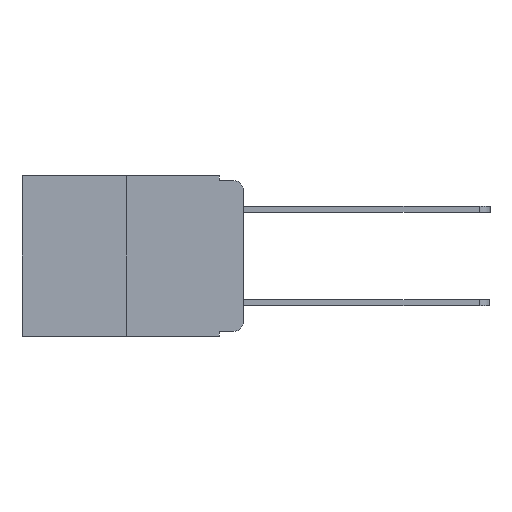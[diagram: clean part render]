
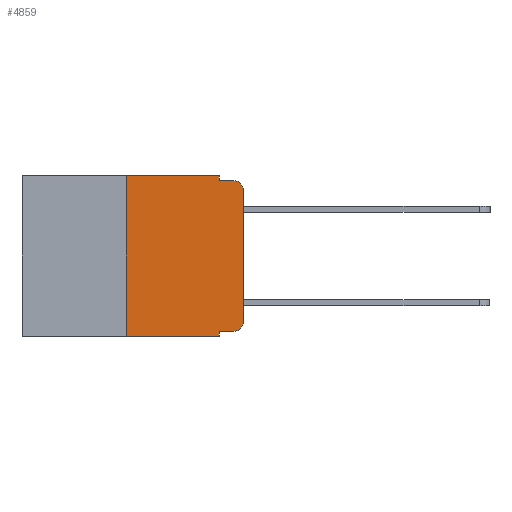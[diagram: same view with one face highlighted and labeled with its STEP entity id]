
A CAD part, left-side view. The second image highlights one B-rep face of the part: STEP entity #4859.
In plain terms, the highlighted planar face has unit normal (-1, 0, 0).
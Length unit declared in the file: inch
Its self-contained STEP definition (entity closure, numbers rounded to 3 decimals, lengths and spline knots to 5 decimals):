
#350 = VERTEX_POINT ( 'NONE', #8373 ) ;
#452 = LINE ( 'NONE', #888, #8284 ) ;
#463 = DIRECTION ( 'NONE',  ( 0., 0., -1. ) ) ;
#888 = CARTESIAN_POINT ( 'NONE',  ( 0., 0.473, -0.343 ) ) ;
#936 = CARTESIAN_POINT ( 'NONE',  ( 0., 0.051, -0.333 ) ) ;
#1066 = ORIENTED_EDGE ( 'NONE', *, *, #5062, .F. ) ;
#1341 = CIRCLE ( 'NONE', #8610, 0.02 ) ;
#1347 = PLANE ( 'NONE',  #12358 ) ;
#1623 = LINE ( 'NONE', #2709, #12249 ) ;
#1631 = CARTESIAN_POINT ( 'NONE',  ( 0., 0.02, -0.333 ) ) ;
#1975 = EDGE_CURVE ( 'NONE', #10013, #10409, #1341, .T. ) ;
#2271 = LINE ( 'NONE', #11626, #12430 ) ;
#2469 = CARTESIAN_POINT ( 'NONE',  ( 0., 0.02, -0.03 ) ) ;
#2486 = VECTOR ( 'NONE', #4466, 39.37008 ) ;
#2709 = CARTESIAN_POINT ( 'NONE',  ( 0., 0.25, 0. ) ) ;
#2778 = EDGE_CURVE ( 'NONE', #6278, #10013, #9922, .T. ) ;
#3010 = ORIENTED_EDGE ( 'NONE', *, *, #7052, .T. ) ;
#3374 = DIRECTION ( 'NONE',  ( 0., -1., 0. ) ) ;
#3494 = ORIENTED_EDGE ( 'NONE', *, *, #8105, .T. ) ;
#3567 = EDGE_CURVE ( 'NONE', #6278, #4012, #2271, .T. ) ;
#3633 = DIRECTION ( 'NONE',  ( 0., 0., -1. ) ) ;
#3638 = DIRECTION ( 'NONE',  ( 0., 0., -1. ) ) ;
#3853 = DIRECTION ( 'NONE',  ( 0., -1., 0. ) ) ;
#3870 = ORIENTED_EDGE ( 'NONE', *, *, #1975, .T. ) ;
#3961 = VECTOR ( 'NONE', #3853, 39.37008 ) ;
#4004 = CARTESIAN_POINT ( 'NONE',  ( 0., 0.051, -0.333 ) ) ;
#4012 = VERTEX_POINT ( 'NONE', #10223 ) ;
#4240 = EDGE_CURVE ( 'NONE', #5392, #350, #13506, .T. ) ;
#4338 = EDGE_CURVE ( 'NONE', #12383, #5392, #1623, .T. ) ;
#4466 = DIRECTION ( 'NONE',  ( 0., 0., 1. ) ) ;
#4538 = CARTESIAN_POINT ( 'NONE',  ( 0., 0.25, -0.343 ) ) ;
#4859 = ADVANCED_FACE ( 'NONE', ( #8910 ), #1347, .F. ) ;
#4999 = DIRECTION ( 'NONE',  ( 0., 0., 1. ) ) ;
#5062 = EDGE_CURVE ( 'NONE', #350, #11182, #11923, .T. ) ;
#5392 = VERTEX_POINT ( 'NONE', #8377 ) ;
#5452 = LINE ( 'NONE', #11368, #2486 ) ;
#5738 = EDGE_CURVE ( 'NONE', #11182, #8103, #9769, .T. ) ;
#5886 = CARTESIAN_POINT ( 'NONE',  ( 0., 0.473, 0. ) ) ;
#5915 = DIRECTION ( 'NONE',  ( 0., 0., -1. ) ) ;
#5934 = ORIENTED_EDGE ( 'NONE', *, *, #6382, .T. ) ;
#6021 = DIRECTION ( 'NONE',  ( -1., 0., 0. ) ) ;
#6278 = VERTEX_POINT ( 'NONE', #936 ) ;
#6300 = ORIENTED_EDGE ( 'NONE', *, *, #2778, .T. ) ;
#6382 = EDGE_CURVE ( 'NONE', #7345, #8103, #13264, .T. ) ;
#6808 = ORIENTED_EDGE ( 'NONE', *, *, #4338, .F. ) ;
#6817 = CARTESIAN_POINT ( 'NONE',  ( 0., 0., -0.03 ) ) ;
#7052 = EDGE_CURVE ( 'NONE', #10409, #7345, #5452, .T. ) ;
#7263 = ORIENTED_EDGE ( 'NONE', *, *, #4240, .F. ) ;
#7345 = VERTEX_POINT ( 'NONE', #6817 ) ;
#8103 = VERTEX_POINT ( 'NONE', #13322 ) ;
#8105 = EDGE_CURVE ( 'NONE', #12383, #4012, #452, .T. ) ;
#8147 = AXIS2_PLACEMENT_3D ( 'NONE', #2469, #9712, #3638 ) ;
#8284 = VECTOR ( 'NONE', #3374, 39.37008 ) ;
#8373 = CARTESIAN_POINT ( 'NONE',  ( 0., 0.051, 0. ) ) ;
#8377 = CARTESIAN_POINT ( 'NONE',  ( 0., 0.25, 0. ) ) ;
#8610 = AXIS2_PLACEMENT_3D ( 'NONE', #11833, #6021, #12823 ) ;
#8658 = CARTESIAN_POINT ( 'NONE',  ( 0., 0., -0.313 ) ) ;
#8910 = FACE_OUTER_BOUND ( 'NONE', #10729, .T. ) ;
#9351 = ORIENTED_EDGE ( 'NONE', *, *, #3567, .F. ) ;
#9361 = VECTOR ( 'NONE', #463, 39.37008 ) ;
#9456 = ORIENTED_EDGE ( 'NONE', *, *, #5738, .F. ) ;
#9462 = CARTESIAN_POINT ( 'NONE',  ( 0., 0.051, -0.01 ) ) ;
#9712 = DIRECTION ( 'NONE',  ( -1., 0., 0. ) ) ;
#9769 = LINE ( 'NONE', #10856, #3961 ) ;
#9812 = CARTESIAN_POINT ( 'NONE',  ( 0., 0.473, 0. ) ) ;
#9922 = LINE ( 'NONE', #4004, #10235 ) ;
#10013 = VERTEX_POINT ( 'NONE', #1631 ) ;
#10223 = CARTESIAN_POINT ( 'NONE',  ( 0., 0.051, -0.343 ) ) ;
#10235 = VECTOR ( 'NONE', #10986, 39.37008 ) ;
#10409 = VERTEX_POINT ( 'NONE', #8658 ) ;
#10729 = EDGE_LOOP ( 'NONE', ( #3010, #5934, #9456, #1066, #7263, #6808, #3494, #9351, #6300, #3870 ) ) ;
#10856 = CARTESIAN_POINT ( 'NONE',  ( 0., 0.051, -0.01 ) ) ;
#10986 = DIRECTION ( 'NONE',  ( 0., -1., 0. ) ) ;
#11064 = CARTESIAN_POINT ( 'NONE',  ( 0., 0.051, 0. ) ) ;
#11182 = VERTEX_POINT ( 'NONE', #9462 ) ;
#11368 = CARTESIAN_POINT ( 'NONE',  ( 0., 0., 0. ) ) ;
#11626 = CARTESIAN_POINT ( 'NONE',  ( 0., 0.051, 0. ) ) ;
#11731 = DIRECTION ( 'NONE',  ( 1., 0., 0. ) ) ;
#11833 = CARTESIAN_POINT ( 'NONE',  ( 0., 0.02, -0.313 ) ) ;
#11923 = LINE ( 'NONE', #11064, #9361 ) ;
#12249 = VECTOR ( 'NONE', #4999, 39.37008 ) ;
#12358 = AXIS2_PLACEMENT_3D ( 'NONE', #9812, #11731, #5915 ) ;
#12383 = VERTEX_POINT ( 'NONE', #4538 ) ;
#12430 = VECTOR ( 'NONE', #3633, 39.37008 ) ;
#12680 = DIRECTION ( 'NONE',  ( 0., -1., 0. ) ) ;
#12823 = DIRECTION ( 'NONE',  ( 0., 0., -1. ) ) ;
#13195 = VECTOR ( 'NONE', #12680, 39.37008 ) ;
#13264 = CIRCLE ( 'NONE', #8147, 0.02 ) ;
#13322 = CARTESIAN_POINT ( 'NONE',  ( 0., 0.02, -0.01 ) ) ;
#13506 = LINE ( 'NONE', #5886, #13195 ) ;
